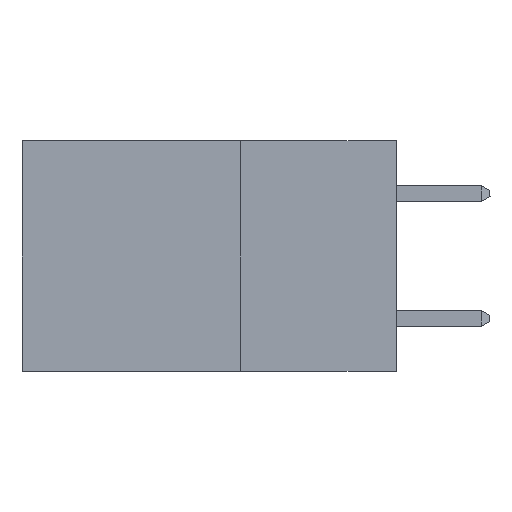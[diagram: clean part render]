
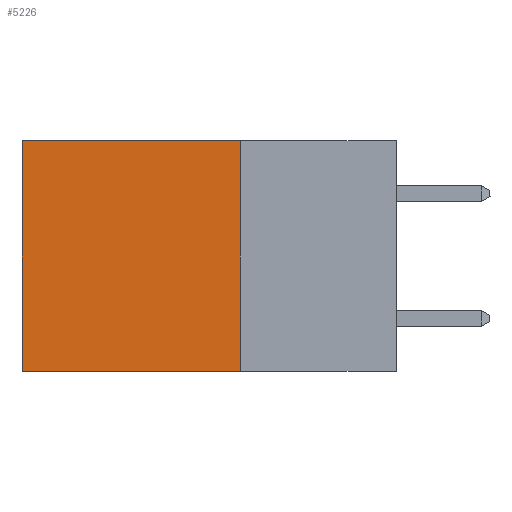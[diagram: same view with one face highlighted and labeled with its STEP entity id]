
A CAD part, left-side view. The second image highlights one B-rep face of the part: STEP entity #5226.
In plain terms, the highlighted planar face has unit normal (-1, 0, 0).
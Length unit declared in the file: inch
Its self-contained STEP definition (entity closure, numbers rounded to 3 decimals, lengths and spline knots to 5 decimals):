
#2579 = VERTEX_POINT ( 'NONE', #5182 ) ;
#3786 = LINE ( 'NONE', #10214, #17063 ) ;
#3864 = ORIENTED_EDGE ( 'NONE', *, *, #18161, .T. ) ;
#4715 = DIRECTION ( 'NONE',  ( 0., 0., -1. ) ) ;
#4740 = DIRECTION ( 'NONE',  ( 1., 0., 0. ) ) ;
#4808 = PLANE ( 'NONE',  #9881 ) ;
#5182 = CARTESIAN_POINT ( 'NONE',  ( 0.2615, 0.6, 0. ) ) ;
#5226 = ADVANCED_FACE ( 'NONE', ( #16466 ), #4808, .F. ) ;
#5234 = CARTESIAN_POINT ( 'NONE',  ( 0.2615, 0.25, -0.37 ) ) ;
#6095 = DIRECTION ( 'NONE',  ( 0., 1., 0. ) ) ;
#6123 = VERTEX_POINT ( 'NONE', #18105 ) ;
#6177 = VECTOR ( 'NONE', #14953, 39.37008 ) ;
#8611 = DIRECTION ( 'NONE',  ( 0., 0., -1. ) ) ;
#8741 = ORIENTED_EDGE ( 'NONE', *, *, #18526, .F. ) ;
#9013 = CARTESIAN_POINT ( 'NONE',  ( 0.2615, 0.25, -0.37 ) ) ;
#9186 = VERTEX_POINT ( 'NONE', #9013 ) ;
#9793 = CARTESIAN_POINT ( 'NONE',  ( 0.2615, 0.25, 0. ) ) ;
#9881 = AXIS2_PLACEMENT_3D ( 'NONE', #5234, #4740, #4715 ) ;
#10214 = CARTESIAN_POINT ( 'NONE',  ( 0.2615, 0.6, -0.37 ) ) ;
#11227 = CARTESIAN_POINT ( 'NONE',  ( 0.2615, 0.25, 0. ) ) ;
#11722 = LINE ( 'NONE', #11227, #15816 ) ;
#12844 = ORIENTED_EDGE ( 'NONE', *, *, #20723, .T. ) ;
#13886 = EDGE_LOOP ( 'NONE', ( #12844, #8741, #15942, #3864 ) ) ;
#14953 = DIRECTION ( 'NONE',  ( 0., 0., -1. ) ) ;
#15340 = LINE ( 'NONE', #16687, #6177 ) ;
#15816 = VECTOR ( 'NONE', #6095, 39.37008 ) ;
#15942 = ORIENTED_EDGE ( 'NONE', *, *, #16854, .F. ) ;
#16466 = FACE_OUTER_BOUND ( 'NONE', #13886, .T. ) ;
#16687 = CARTESIAN_POINT ( 'NONE',  ( 0.2615, 0.25, -0.37 ) ) ;
#16854 = EDGE_CURVE ( 'NONE', #21825, #9186, #15340, .T. ) ;
#17063 = VECTOR ( 'NONE', #8611, 39.37008 ) ;
#17285 = CARTESIAN_POINT ( 'NONE',  ( 0.2615, 0.25, -0.37 ) ) ;
#18105 = CARTESIAN_POINT ( 'NONE',  ( 0.2615, 0.6, -0.37 ) ) ;
#18161 = EDGE_CURVE ( 'NONE', #21825, #2579, #11722, .T. ) ;
#18526 = EDGE_CURVE ( 'NONE', #9186, #6123, #21882, .T. ) ;
#20723 = EDGE_CURVE ( 'NONE', #2579, #6123, #3786, .T. ) ;
#21379 = VECTOR ( 'NONE', #22359, 39.37008 ) ;
#21825 = VERTEX_POINT ( 'NONE', #9793 ) ;
#21882 = LINE ( 'NONE', #17285, #21379 ) ;
#22359 = DIRECTION ( 'NONE',  ( 0., 1., 0. ) ) ;
